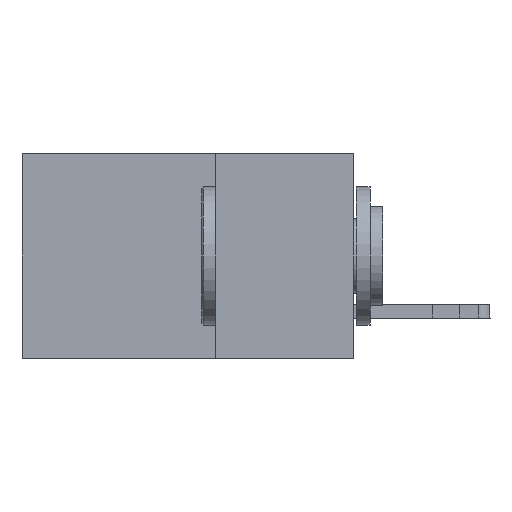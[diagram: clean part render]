
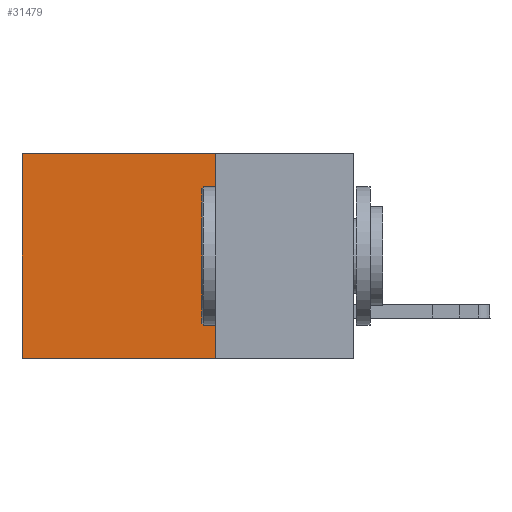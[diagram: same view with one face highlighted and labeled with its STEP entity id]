
A CAD part, left-side view. The second image highlights one B-rep face of the part: STEP entity #31479.
In plain terms, the highlighted planar face has unit normal (-1, 0, 0).
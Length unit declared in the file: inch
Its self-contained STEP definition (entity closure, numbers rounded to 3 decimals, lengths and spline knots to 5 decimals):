
#679 = CARTESIAN_POINT ( 'NONE',  ( 0.2875, 0.25, 0. ) ) ;
#812 = LINE ( 'NONE', #21511, #7959 ) ;
#1172 = ORIENTED_EDGE ( 'NONE', *, *, #25345, .T. ) ;
#1528 = VECTOR ( 'NONE', #2089, 39.37008 ) ;
#2089 = DIRECTION ( 'NONE',  ( 0., 1., 0. ) ) ;
#3948 = CARTESIAN_POINT ( 'NONE',  ( 0.2875, 0.25, 0. ) ) ;
#4467 = ORIENTED_EDGE ( 'NONE', *, *, #8903, .F. ) ;
#7959 = VECTOR ( 'NONE', #19488, 39.37008 ) ;
#8601 = CARTESIAN_POINT ( 'NONE',  ( 0.2875, 0.6, -0.37 ) ) ;
#8903 = EDGE_CURVE ( 'NONE', #15331, #28267, #26665, .T. ) ;
#10701 = VERTEX_POINT ( 'NONE', #22954 ) ;
#12484 = EDGE_CURVE ( 'NONE', #25975, #15331, #812, .T. ) ;
#12880 = CARTESIAN_POINT ( 'NONE',  ( 0.2875, 0.25, -0.37 ) ) ;
#14162 = DIRECTION ( 'NONE',  ( 0., 1., 0. ) ) ;
#14810 = CARTESIAN_POINT ( 'NONE',  ( 0.2875, 0.25, 0. ) ) ;
#15331 = VERTEX_POINT ( 'NONE', #12880 ) ;
#16987 = CARTESIAN_POINT ( 'NONE',  ( 0.2875, 0.25, -0.37 ) ) ;
#17941 = AXIS2_PLACEMENT_3D ( 'NONE', #14810, #30951, #33259 ) ;
#19488 = DIRECTION ( 'NONE',  ( 0., 0., -1. ) ) ;
#19810 = VECTOR ( 'NONE', #23994, 39.37008 ) ;
#20223 = LINE ( 'NONE', #679, #30198 ) ;
#21511 = CARTESIAN_POINT ( 'NONE',  ( 0.2875, 0.25, 0. ) ) ;
#22954 = CARTESIAN_POINT ( 'NONE',  ( 0.2875, 0.6, 0. ) ) ;
#23068 = ORIENTED_EDGE ( 'NONE', *, *, #12484, .F. ) ;
#23665 = CARTESIAN_POINT ( 'NONE',  ( 0.2875, 0.6, 0. ) ) ;
#23994 = DIRECTION ( 'NONE',  ( 0., 0., -1. ) ) ;
#25345 = EDGE_CURVE ( 'NONE', #25975, #10701, #20223, .T. ) ;
#25553 = FACE_OUTER_BOUND ( 'NONE', #32247, .T. ) ;
#25975 = VERTEX_POINT ( 'NONE', #3948 ) ;
#26490 = LINE ( 'NONE', #23665, #19810 ) ;
#26665 = LINE ( 'NONE', #16987, #1528 ) ;
#28140 = PLANE ( 'NONE',  #17941 ) ;
#28267 = VERTEX_POINT ( 'NONE', #8601 ) ;
#30198 = VECTOR ( 'NONE', #14162, 39.37008 ) ;
#30238 = ORIENTED_EDGE ( 'NONE', *, *, #30683, .T. ) ;
#30683 = EDGE_CURVE ( 'NONE', #10701, #28267, #26490, .T. ) ;
#30951 = DIRECTION ( 'NONE',  ( 1., 0., 0. ) ) ;
#31479 = ADVANCED_FACE ( 'NONE', ( #25553 ), #28140, .F. ) ;
#32247 = EDGE_LOOP ( 'NONE', ( #30238, #4467, #23068, #1172 ) ) ;
#33259 = DIRECTION ( 'NONE',  ( 0., 0., -1. ) ) ;
